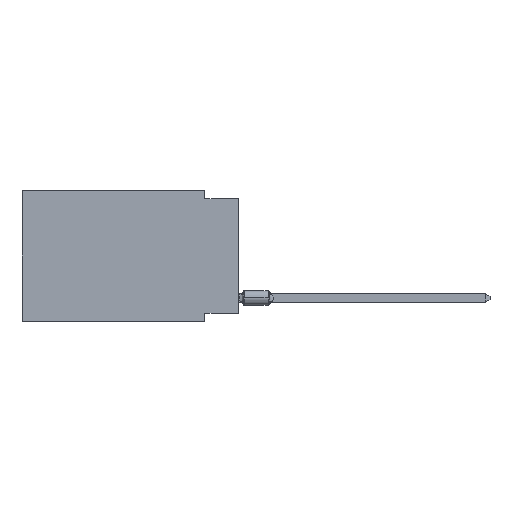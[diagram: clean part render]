
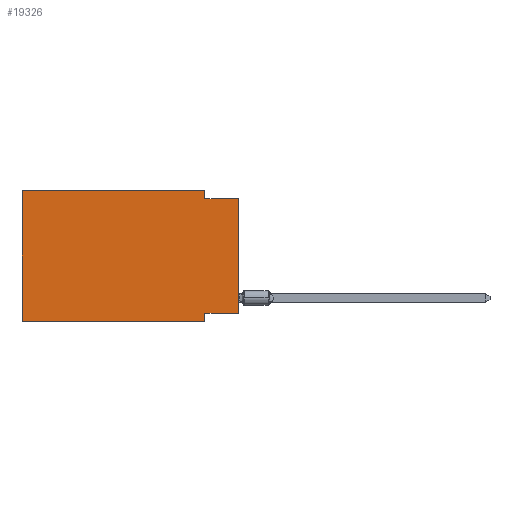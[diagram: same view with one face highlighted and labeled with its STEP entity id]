
A CAD part, left-side view. The second image highlights one B-rep face of the part: STEP entity #19326.
In plain terms, the highlighted planar face has unit normal (-1, 0, 0).
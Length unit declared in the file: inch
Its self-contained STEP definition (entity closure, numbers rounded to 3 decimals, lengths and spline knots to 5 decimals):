
#15 = CARTESIAN_POINT ( 'NONE',  ( 0., 0.645, 0. ) ) ;
#411 = LINE ( 'NONE', #9930, #7319 ) ;
#866 = LINE ( 'NONE', #8736, #13988 ) ;
#948 = AXIS2_PLACEMENT_3D ( 'NONE', #15, #5866, #6110 ) ;
#953 = CARTESIAN_POINT ( 'NONE',  ( 0., 0.1, 0. ) ) ;
#1256 = VERTEX_POINT ( 'NONE', #3377 ) ;
#1515 = CARTESIAN_POINT ( 'NONE',  ( 0., 0.645, 0. ) ) ;
#2041 = EDGE_CURVE ( 'NONE', #1256, #15143, #16844, .T. ) ;
#2518 = LINE ( 'NONE', #19168, #7376 ) ;
#2620 = ORIENTED_EDGE ( 'NONE', *, *, #21005, .F. ) ;
#2660 = CARTESIAN_POINT ( 'NONE',  ( 0., 0.645, 0. ) ) ;
#2868 = CARTESIAN_POINT ( 'NONE',  ( 0., 0., 0. ) ) ;
#3241 = DIRECTION ( 'NONE',  ( 0., 0., 1. ) ) ;
#3377 = CARTESIAN_POINT ( 'NONE',  ( 0., 0.645, 0. ) ) ;
#4700 = DIRECTION ( 'NONE',  ( 0., 0., -1. ) ) ;
#5299 = DIRECTION ( 'NONE',  ( 0., -1., 0. ) ) ;
#5753 = ORIENTED_EDGE ( 'NONE', *, *, #13987, .F. ) ;
#5866 = DIRECTION ( 'NONE',  ( 1., 0., 0. ) ) ;
#6110 = DIRECTION ( 'NONE',  ( 0., 0., -1. ) ) ;
#6613 = CARTESIAN_POINT ( 'NONE',  ( 0., 0.645, -0.39 ) ) ;
#7272 = VERTEX_POINT ( 'NONE', #8731 ) ;
#7319 = VECTOR ( 'NONE', #10047, 39.37008 ) ;
#7376 = VECTOR ( 'NONE', #17255, 39.37008 ) ;
#8029 = LINE ( 'NONE', #19461, #12298 ) ;
#8578 = VERTEX_POINT ( 'NONE', #6613 ) ;
#8731 = CARTESIAN_POINT ( 'NONE',  ( 0., 0.1, -0.39 ) ) ;
#8736 = CARTESIAN_POINT ( 'NONE',  ( 0., 0., -0.365 ) ) ;
#8788 = VECTOR ( 'NONE', #5299, 39.37008 ) ;
#9526 = VERTEX_POINT ( 'NONE', #11198 ) ;
#9930 = CARTESIAN_POINT ( 'NONE',  ( 0., 0.645, -0.39 ) ) ;
#10047 = DIRECTION ( 'NONE',  ( 0., -1., 0. ) ) ;
#11198 = CARTESIAN_POINT ( 'NONE',  ( 0., 0., -0.025 ) ) ;
#11316 = ORIENTED_EDGE ( 'NONE', *, *, #11933, .T. ) ;
#11933 = EDGE_CURVE ( 'NONE', #14981, #9526, #22163, .T. ) ;
#11946 = FACE_OUTER_BOUND ( 'NONE', #18551, .T. ) ;
#12278 = EDGE_CURVE ( 'NONE', #8578, #7272, #411, .T. ) ;
#12298 = VECTOR ( 'NONE', #13867, 39.37008 ) ;
#12525 = DIRECTION ( 'NONE',  ( 0., 1., 0. ) ) ;
#12586 = VERTEX_POINT ( 'NONE', #23391 ) ;
#12796 = LINE ( 'NONE', #24374, #13495 ) ;
#12871 = DIRECTION ( 'NONE',  ( 0., 0., 1. ) ) ;
#13495 = VECTOR ( 'NONE', #4700, 39.37008 ) ;
#13867 = DIRECTION ( 'NONE',  ( 0., 0., -1. ) ) ;
#13987 = EDGE_CURVE ( 'NONE', #18497, #9526, #2518, .T. ) ;
#13988 = VECTOR ( 'NONE', #12525, 39.37008 ) ;
#14981 = VERTEX_POINT ( 'NONE', #15661 ) ;
#15143 = VERTEX_POINT ( 'NONE', #953 ) ;
#15661 = CARTESIAN_POINT ( 'NONE',  ( 0., 0., -0.365 ) ) ;
#15884 = ORIENTED_EDGE ( 'NONE', *, *, #23294, .F. ) ;
#16844 = LINE ( 'NONE', #1515, #8788 ) ;
#17255 = DIRECTION ( 'NONE',  ( 0., -1., 0. ) ) ;
#17399 = PLANE ( 'NONE',  #948 ) ;
#17773 = ORIENTED_EDGE ( 'NONE', *, *, #12278, .T. ) ;
#18497 = VERTEX_POINT ( 'NONE', #22730 ) ;
#18551 = EDGE_LOOP ( 'NONE', ( #11316, #5753, #2620, #22183, #21955, #17773, #18734, #15884 ) ) ;
#18734 = ORIENTED_EDGE ( 'NONE', *, *, #21498, .F. ) ;
#19065 = VECTOR ( 'NONE', #3241, 39.37008 ) ;
#19168 = CARTESIAN_POINT ( 'NONE',  ( 0., 0., -0.025 ) ) ;
#19326 = ADVANCED_FACE ( 'NONE', ( #11946 ), #17399, .F. ) ;
#19461 = CARTESIAN_POINT ( 'NONE',  ( 0., 0.1, -0.39 ) ) ;
#21005 = EDGE_CURVE ( 'NONE', #15143, #18497, #12796, .T. ) ;
#21498 = EDGE_CURVE ( 'NONE', #12586, #7272, #8029, .T. ) ;
#21955 = ORIENTED_EDGE ( 'NONE', *, *, #22161, .F. ) ;
#22161 = EDGE_CURVE ( 'NONE', #8578, #1256, #22664, .T. ) ;
#22163 = LINE ( 'NONE', #2868, #19065 ) ;
#22183 = ORIENTED_EDGE ( 'NONE', *, *, #2041, .F. ) ;
#22664 = LINE ( 'NONE', #2660, #22890 ) ;
#22730 = CARTESIAN_POINT ( 'NONE',  ( 0., 0.1, -0.025 ) ) ;
#22890 = VECTOR ( 'NONE', #12871, 39.37008 ) ;
#23294 = EDGE_CURVE ( 'NONE', #14981, #12586, #866, .T. ) ;
#23391 = CARTESIAN_POINT ( 'NONE',  ( 0., 0.1, -0.365 ) ) ;
#24374 = CARTESIAN_POINT ( 'NONE',  ( 0., 0.1, 0. ) ) ;
